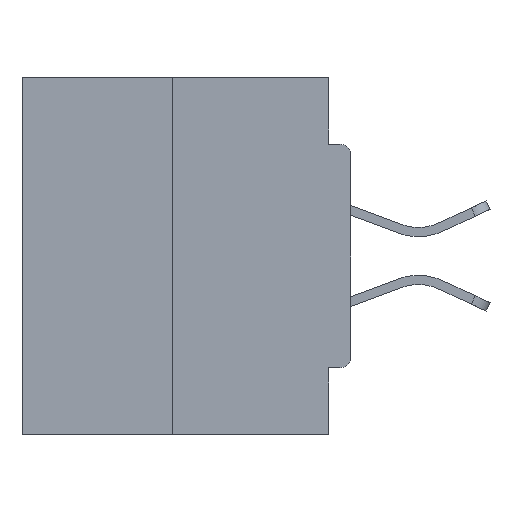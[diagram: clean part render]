
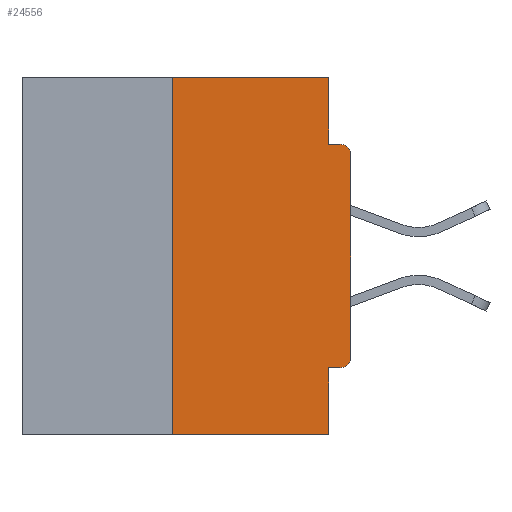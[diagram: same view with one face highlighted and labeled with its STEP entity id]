
A CAD part, left-side view. The second image highlights one B-rep face of the part: STEP entity #24556.
In plain terms, the highlighted planar face has unit normal (-1, 0, 0).
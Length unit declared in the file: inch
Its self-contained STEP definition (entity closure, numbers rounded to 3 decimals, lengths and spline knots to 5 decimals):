
#358 = VERTEX_POINT ( 'NONE', #16085 ) ;
#490 = CARTESIAN_POINT ( 'NONE',  ( 0., 0.015, -0.3915 ) ) ;
#617 = ORIENTED_EDGE ( 'NONE', *, *, #28861, .T. ) ;
#1487 = AXIS2_PLACEMENT_3D ( 'NONE', #34817, #23903, #1861 ) ;
#1861 = DIRECTION ( 'NONE',  ( 0., 0., -1. ) ) ;
#2390 = CARTESIAN_POINT ( 'NONE',  ( 0., 0., 0. ) ) ;
#2713 = CARTESIAN_POINT ( 'NONE',  ( 0., 0.031, 0. ) ) ;
#3114 = VERTEX_POINT ( 'NONE', #3446 ) ;
#3446 = CARTESIAN_POINT ( 'NONE',  ( 0., 0.031, -0.5 ) ) ;
#4761 = EDGE_CURVE ( 'NONE', #34456, #19938, #13415, .T. ) ;
#5499 = ORIENTED_EDGE ( 'NONE', *, *, #8651, .T. ) ;
#6357 = CARTESIAN_POINT ( 'NONE',  ( 0., 0.031, 0. ) ) ;
#6982 = DIRECTION ( 'NONE',  ( 0., -1., 0. ) ) ;
#7246 = CARTESIAN_POINT ( 'NONE',  ( 0., 0.015, -0.0935 ) ) ;
#7671 = PLANE ( 'NONE',  #1487 ) ;
#8540 = DIRECTION ( 'NONE',  ( -1., 0., 0. ) ) ;
#8651 = EDGE_CURVE ( 'NONE', #34456, #358, #16079, .T. ) ;
#8713 = CARTESIAN_POINT ( 'NONE',  ( 0., 0., -0.0935 ) ) ;
#8767 = EDGE_CURVE ( 'NONE', #24171, #32675, #14417, .T. ) ;
#10210 = ORIENTED_EDGE ( 'NONE', *, *, #13174, .F. ) ;
#10227 = DIRECTION ( 'NONE',  ( 0., 0., 1. ) ) ;
#10288 = CARTESIAN_POINT ( 'NONE',  ( 0., 0.46, 0. ) ) ;
#10486 = VECTOR ( 'NONE', #16267, 39.37008 ) ;
#10913 = DIRECTION ( 'NONE',  ( 0., 0., -1. ) ) ;
#12290 = EDGE_CURVE ( 'NONE', #19938, #3114, #15962, .T. ) ;
#12681 = CARTESIAN_POINT ( 'NONE',  ( 0., 0.015, -0.1085 ) ) ;
#13174 = EDGE_CURVE ( 'NONE', #18624, #15812, #17620, .T. ) ;
#13415 = LINE ( 'NONE', #26956, #10486 ) ;
#13457 = AXIS2_PLACEMENT_3D ( 'NONE', #490, #8540, #16811 ) ;
#13570 = VECTOR ( 'NONE', #16927, 39.37008 ) ;
#14386 = VERTEX_POINT ( 'NONE', #25729 ) ;
#14394 = EDGE_CURVE ( 'NONE', #24171, #3114, #30719, .T. ) ;
#14417 = LINE ( 'NONE', #30576, #13570 ) ;
#14583 = CARTESIAN_POINT ( 'NONE',  ( 0., 0.031, -0.4065 ) ) ;
#15711 = VECTOR ( 'NONE', #24015, 39.37008 ) ;
#15812 = VERTEX_POINT ( 'NONE', #24527 ) ;
#15962 = LINE ( 'NONE', #21414, #19805 ) ;
#16079 = CIRCLE ( 'NONE', #13457, 0.015 ) ;
#16085 = CARTESIAN_POINT ( 'NONE',  ( 0., 0., -0.3915 ) ) ;
#16267 = DIRECTION ( 'NONE',  ( 0., 1., 0. ) ) ;
#16366 = EDGE_CURVE ( 'NONE', #15812, #34824, #28400, .T. ) ;
#16811 = DIRECTION ( 'NONE',  ( 0., 0., -1. ) ) ;
#16927 = DIRECTION ( 'NONE',  ( 0., 0., 1. ) ) ;
#17239 = ORIENTED_EDGE ( 'NONE', *, *, #4761, .F. ) ;
#17620 = LINE ( 'NONE', #2713, #28645 ) ;
#18089 = CARTESIAN_POINT ( 'NONE',  ( 0., 0.25, 0. ) ) ;
#18414 = CIRCLE ( 'NONE', #25150, 0.015 ) ;
#18624 = VERTEX_POINT ( 'NONE', #6357 ) ;
#19805 = VECTOR ( 'NONE', #26850, 39.37008 ) ;
#19938 = VERTEX_POINT ( 'NONE', #14583 ) ;
#20202 = FACE_OUTER_BOUND ( 'NONE', #33044, .T. ) ;
#20729 = ORIENTED_EDGE ( 'NONE', *, *, #27245, .F. ) ;
#21414 = CARTESIAN_POINT ( 'NONE',  ( 0., 0.031, -0.5 ) ) ;
#22948 = LINE ( 'NONE', #10288, #15711 ) ;
#23232 = CARTESIAN_POINT ( 'NONE',  ( 0., 0.46, -0.5 ) ) ;
#23903 = DIRECTION ( 'NONE',  ( 1., 0., 0. ) ) ;
#24015 = DIRECTION ( 'NONE',  ( 0., -1., 0. ) ) ;
#24091 = LINE ( 'NONE', #2390, #28768 ) ;
#24133 = VECTOR ( 'NONE', #30520, 39.37008 ) ;
#24171 = VERTEX_POINT ( 'NONE', #31242 ) ;
#24527 = CARTESIAN_POINT ( 'NONE',  ( 0., 0.031, -0.0935 ) ) ;
#24556 = ADVANCED_FACE ( 'NONE', ( #20202 ), #7671, .F. ) ;
#25150 = AXIS2_PLACEMENT_3D ( 'NONE', #12681, #31755, #34482 ) ;
#25729 = CARTESIAN_POINT ( 'NONE',  ( 0., 0., -0.1085 ) ) ;
#26050 = VECTOR ( 'NONE', #6982, 39.37008 ) ;
#26850 = DIRECTION ( 'NONE',  ( 0., 0., -1. ) ) ;
#26956 = CARTESIAN_POINT ( 'NONE',  ( 0., 0., -0.4065 ) ) ;
#27245 = EDGE_CURVE ( 'NONE', #32675, #18624, #22948, .T. ) ;
#28400 = LINE ( 'NONE', #8713, #24133 ) ;
#28645 = VECTOR ( 'NONE', #10913, 39.37008 ) ;
#28768 = VECTOR ( 'NONE', #10227, 39.37008 ) ;
#28861 = EDGE_CURVE ( 'NONE', #14386, #34824, #18414, .T. ) ;
#28991 = ORIENTED_EDGE ( 'NONE', *, *, #8767, .F. ) ;
#30520 = DIRECTION ( 'NONE',  ( 0., -1., 0. ) ) ;
#30576 = CARTESIAN_POINT ( 'NONE',  ( 0., 0.25, 0. ) ) ;
#30719 = LINE ( 'NONE', #23232, #26050 ) ;
#31242 = CARTESIAN_POINT ( 'NONE',  ( 0., 0.25, -0.5 ) ) ;
#31454 = ORIENTED_EDGE ( 'NONE', *, *, #14394, .T. ) ;
#31755 = DIRECTION ( 'NONE',  ( -1., 0., 0. ) ) ;
#32471 = ORIENTED_EDGE ( 'NONE', *, *, #16366, .F. ) ;
#32577 = EDGE_CURVE ( 'NONE', #358, #14386, #24091, .T. ) ;
#32675 = VERTEX_POINT ( 'NONE', #18089 ) ;
#33044 = EDGE_LOOP ( 'NONE', ( #20729, #28991, #31454, #34644, #17239, #5499, #33544, #617, #32471, #10210 ) ) ;
#33289 = CARTESIAN_POINT ( 'NONE',  ( 0., 0.015, -0.4065 ) ) ;
#33544 = ORIENTED_EDGE ( 'NONE', *, *, #32577, .T. ) ;
#34456 = VERTEX_POINT ( 'NONE', #33289 ) ;
#34482 = DIRECTION ( 'NONE',  ( 0., 0., -1. ) ) ;
#34644 = ORIENTED_EDGE ( 'NONE', *, *, #12290, .F. ) ;
#34817 = CARTESIAN_POINT ( 'NONE',  ( 0., 0.46, 0. ) ) ;
#34824 = VERTEX_POINT ( 'NONE', #7246 ) ;
